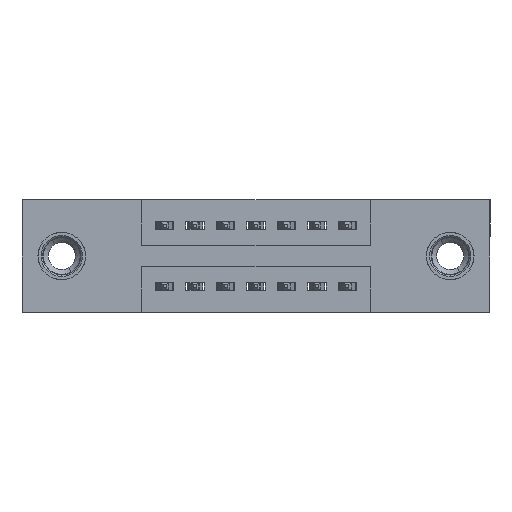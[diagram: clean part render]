
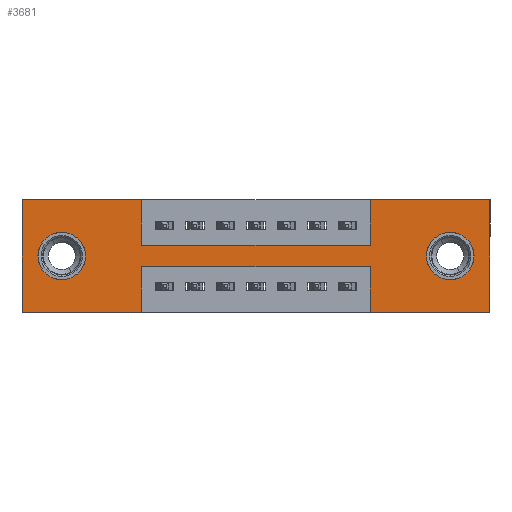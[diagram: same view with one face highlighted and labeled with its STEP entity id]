
A CAD part, front view. The second image highlights one B-rep face of the part: STEP entity #3681.
In plain terms, the highlighted planar face has unit normal (0, -1, 0).
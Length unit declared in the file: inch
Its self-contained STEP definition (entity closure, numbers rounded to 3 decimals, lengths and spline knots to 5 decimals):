
#15 = VERTEX_POINT ( 'NONE', #10215 ) ;
#115 = DIRECTION ( 'NONE',  ( 0., 0., -1. ) ) ;
#217 = ORIENTED_EDGE ( 'NONE', *, *, #5495, .T. ) ;
#316 = VERTEX_POINT ( 'NONE', #10917 ) ;
#375 = CARTESIAN_POINT ( 'NONE',  ( 1.405, 0., -0.263 ) ) ;
#463 = CARTESIAN_POINT ( 'NONE',  ( 0., 0., 0. ) ) ;
#607 = VECTOR ( 'NONE', #1782, 39.37008 ) ;
#608 = ORIENTED_EDGE ( 'NONE', *, *, #7334, .F. ) ;
#706 = PLANE ( 'NONE',  #6496 ) ;
#801 = DIRECTION ( 'NONE',  ( -1., 0., 0. ) ) ;
#875 = EDGE_CURVE ( 'NONE', #4007, #15, #11198, .T. ) ;
#892 = VERTEX_POINT ( 'NONE', #3567 ) ;
#929 = LINE ( 'NONE', #3808, #607 ) ;
#1279 = CARTESIAN_POINT ( 'NONE',  ( 0.3925, 0., -0.22 ) ) ;
#1328 = EDGE_LOOP ( 'NONE', ( #2870, #9219 ) ) ;
#1419 = LINE ( 'NONE', #4734, #11276 ) ;
#1485 = VERTEX_POINT ( 'NONE', #4570 ) ;
#1541 = ORIENTED_EDGE ( 'NONE', *, *, #5751, .F. ) ;
#1584 = EDGE_CURVE ( 'NONE', #15, #2349, #8369, .T. ) ;
#1629 = VERTEX_POINT ( 'NONE', #5442 ) ;
#1781 = DIRECTION ( 'NONE',  ( -1., 0., 0. ) ) ;
#1782 = DIRECTION ( 'NONE',  ( 0., 0., -1. ) ) ;
#2278 = EDGE_CURVE ( 'NONE', #892, #4111, #9325, .T. ) ;
#2349 = VERTEX_POINT ( 'NONE', #6331 ) ;
#2431 = VERTEX_POINT ( 'NONE', #5845 ) ;
#2599 = DIRECTION ( 'NONE',  ( 1., 0., 0. ) ) ;
#2659 = LINE ( 'NONE', #9602, #10525 ) ;
#2749 = VERTEX_POINT ( 'NONE', #1279 ) ;
#2765 = CARTESIAN_POINT ( 'NONE',  ( 0., 0., -0.37 ) ) ;
#2800 = DIRECTION ( 'NONE',  ( 0., 0., 1. ) ) ;
#2870 = ORIENTED_EDGE ( 'NONE', *, *, #9489, .T. ) ;
#3197 = EDGE_CURVE ( 'NONE', #8012, #2749, #6570, .T. ) ;
#3241 = CARTESIAN_POINT ( 'NONE',  ( 0.13, 0., -0.185 ) ) ;
#3267 = EDGE_LOOP ( 'NONE', ( #5348, #217 ) ) ;
#3363 = ORIENTED_EDGE ( 'NONE', *, *, #3197, .F. ) ;
#3415 = VECTOR ( 'NONE', #2599, 39.37008 ) ;
#3567 = CARTESIAN_POINT ( 'NONE',  ( 1.405, 0., -0.107 ) ) ;
#3649 = AXIS2_PLACEMENT_3D ( 'NONE', #6778, #6740, #6718 ) ;
#3681 = ADVANCED_FACE ( 'NONE', ( #6557, #6244, #4230 ), #706, .T. ) ;
#3697 = EDGE_CURVE ( 'NONE', #2749, #1485, #929, .T. ) ;
#3753 = AXIS2_PLACEMENT_3D ( 'NONE', #9921, #4281, #10851 ) ;
#3808 = CARTESIAN_POINT ( 'NONE',  ( 0.3925, 0., -0.37 ) ) ;
#4007 = VERTEX_POINT ( 'NONE', #10829 ) ;
#4111 = VERTEX_POINT ( 'NONE', #375 ) ;
#4114 = EDGE_CURVE ( 'NONE', #5319, #4868, #11682, .T. ) ;
#4216 = DIRECTION ( 'NONE',  ( 0., 0., 1. ) ) ;
#4230 = FACE_OUTER_BOUND ( 'NONE', #4938, .T. ) ;
#4281 = DIRECTION ( 'NONE',  ( 0., 1., 0. ) ) ;
#4471 = ORIENTED_EDGE ( 'NONE', *, *, #10329, .F. ) ;
#4570 = CARTESIAN_POINT ( 'NONE',  ( 0.3925, 0., -0.37 ) ) ;
#4626 = ORIENTED_EDGE ( 'NONE', *, *, #875, .F. ) ;
#4734 = CARTESIAN_POINT ( 'NONE',  ( 0., 0., -0.37 ) ) ;
#4776 = CARTESIAN_POINT ( 'NONE',  ( 1.405, 0., -0.185 ) ) ;
#4868 = VERTEX_POINT ( 'NONE', #9271 ) ;
#4908 = DIRECTION ( 'NONE',  ( 0., 0., -1. ) ) ;
#4938 = EDGE_LOOP ( 'NONE', ( #10666, #3363, #4471, #608, #1541, #10652, #8633, #7625, #6540, #11310, #4626, #6871 ) ) ;
#5319 = VERTEX_POINT ( 'NONE', #8257 ) ;
#5348 = ORIENTED_EDGE ( 'NONE', *, *, #2278, .T. ) ;
#5442 = CARTESIAN_POINT ( 'NONE',  ( 0.13, 0., -0.263 ) ) ;
#5495 = EDGE_CURVE ( 'NONE', #4111, #892, #7270, .T. ) ;
#5540 = EDGE_CURVE ( 'NONE', #1485, #4007, #9133, .T. ) ;
#5692 = LINE ( 'NONE', #8409, #3415 ) ;
#5721 = DIRECTION ( 'NONE',  ( 0., 0., -1. ) ) ;
#5751 = EDGE_CURVE ( 'NONE', #4868, #2431, #9526, .T. ) ;
#5774 = DIRECTION ( 'NONE',  ( 0., 0., -1. ) ) ;
#5845 = CARTESIAN_POINT ( 'NONE',  ( 1.535, 0., -0.37 ) ) ;
#6244 = FACE_BOUND ( 'NONE', #1328, .T. ) ;
#6318 = VECTOR ( 'NONE', #7145, 39.37008 ) ;
#6321 = CARTESIAN_POINT ( 'NONE',  ( 0.13, 0., -0.107 ) ) ;
#6331 = CARTESIAN_POINT ( 'NONE',  ( 0.3925, 0., 0. ) ) ;
#6376 = CARTESIAN_POINT ( 'NONE',  ( 0., 0., 0. ) ) ;
#6496 = AXIS2_PLACEMENT_3D ( 'NONE', #2765, #11285, #5721 ) ;
#6540 = ORIENTED_EDGE ( 'NONE', *, *, #9194, .F. ) ;
#6541 = VECTOR ( 'NONE', #9179, 39.37008 ) ;
#6548 = CIRCLE ( 'NONE', #9100, 0.078 ) ;
#6557 = FACE_BOUND ( 'NONE', #3267, .T. ) ;
#6570 = LINE ( 'NONE', #11350, #11141 ) ;
#6718 = DIRECTION ( 'NONE',  ( 0., 0., -1. ) ) ;
#6740 = DIRECTION ( 'NONE',  ( 0., 1., 0. ) ) ;
#6778 = CARTESIAN_POINT ( 'NONE',  ( 1.405, 0., -0.185 ) ) ;
#6788 = VERTEX_POINT ( 'NONE', #7909 ) ;
#6816 = VECTOR ( 'NONE', #115, 39.37008 ) ;
#6871 = ORIENTED_EDGE ( 'NONE', *, *, #5540, .F. ) ;
#7087 = CARTESIAN_POINT ( 'NONE',  ( 1.535, 0., 0. ) ) ;
#7129 = DIRECTION ( 'NONE',  ( 1., 0., 0. ) ) ;
#7145 = DIRECTION ( 'NONE',  ( 0., 0., 1. ) ) ;
#7270 = CIRCLE ( 'NONE', #8255, 0.078 ) ;
#7334 = EDGE_CURVE ( 'NONE', #2431, #11543, #1419, .T. ) ;
#7450 = CARTESIAN_POINT ( 'NONE',  ( 0., 0., 0. ) ) ;
#7596 = EDGE_CURVE ( 'NONE', #1629, #8356, #6548, .T. ) ;
#7609 = CARTESIAN_POINT ( 'NONE',  ( 1.1425, 0., -0.37 ) ) ;
#7625 = ORIENTED_EDGE ( 'NONE', *, *, #10188, .F. ) ;
#7863 = EDGE_CURVE ( 'NONE', #316, #5319, #10398, .T. ) ;
#7909 = CARTESIAN_POINT ( 'NONE',  ( 0.3925, 0., -0.15 ) ) ;
#8012 = VERTEX_POINT ( 'NONE', #9584 ) ;
#8255 = AXIS2_PLACEMENT_3D ( 'NONE', #4776, #11321, #5774 ) ;
#8257 = CARTESIAN_POINT ( 'NONE',  ( 1.1425, 0., 0. ) ) ;
#8356 = VERTEX_POINT ( 'NONE', #6321 ) ;
#8369 = LINE ( 'NONE', #7450, #10752 ) ;
#8409 = CARTESIAN_POINT ( 'NONE',  ( 0.3925, 0., -0.15 ) ) ;
#8482 = DIRECTION ( 'NONE',  ( 0., 0., 1. ) ) ;
#8633 = ORIENTED_EDGE ( 'NONE', *, *, #7863, .F. ) ;
#8960 = VECTOR ( 'NONE', #2800, 39.37008 ) ;
#9100 = AXIS2_PLACEMENT_3D ( 'NONE', #3241, #9862, #4216 ) ;
#9133 = LINE ( 'NONE', #11359, #11532 ) ;
#9179 = DIRECTION ( 'NONE',  ( 1., 0., 0. ) ) ;
#9194 = EDGE_CURVE ( 'NONE', #2349, #6788, #2659, .T. ) ;
#9219 = ORIENTED_EDGE ( 'NONE', *, *, #7596, .T. ) ;
#9227 = LINE ( 'NONE', #12167, #8960 ) ;
#9271 = CARTESIAN_POINT ( 'NONE',  ( 1.535, 0., 0. ) ) ;
#9325 = CIRCLE ( 'NONE', #3649, 0.078 ) ;
#9489 = EDGE_CURVE ( 'NONE', #8356, #1629, #11373, .T. ) ;
#9526 = LINE ( 'NONE', #7087, #6816 ) ;
#9584 = CARTESIAN_POINT ( 'NONE',  ( 1.1425, 0., -0.22 ) ) ;
#9602 = CARTESIAN_POINT ( 'NONE',  ( 0.3925, 0., 0. ) ) ;
#9862 = DIRECTION ( 'NONE',  ( 0., 1., 0. ) ) ;
#9921 = CARTESIAN_POINT ( 'NONE',  ( 0.13, 0., -0.185 ) ) ;
#10104 = VECTOR ( 'NONE', #8482, 39.37008 ) ;
#10188 = EDGE_CURVE ( 'NONE', #6788, #316, #5692, .T. ) ;
#10215 = CARTESIAN_POINT ( 'NONE',  ( 0., 0., 0. ) ) ;
#10259 = CARTESIAN_POINT ( 'NONE',  ( 1.1425, 0., 0. ) ) ;
#10329 = EDGE_CURVE ( 'NONE', #11543, #8012, #9227, .T. ) ;
#10398 = LINE ( 'NONE', #10259, #10104 ) ;
#10525 = VECTOR ( 'NONE', #4908, 39.37008 ) ;
#10652 = ORIENTED_EDGE ( 'NONE', *, *, #4114, .F. ) ;
#10666 = ORIENTED_EDGE ( 'NONE', *, *, #3697, .F. ) ;
#10752 = VECTOR ( 'NONE', #7129, 39.37008 ) ;
#10829 = CARTESIAN_POINT ( 'NONE',  ( 0., 0., -0.37 ) ) ;
#10851 = DIRECTION ( 'NONE',  ( 0., 0., 1. ) ) ;
#10917 = CARTESIAN_POINT ( 'NONE',  ( 1.1425, 0., -0.15 ) ) ;
#11141 = VECTOR ( 'NONE', #11385, 39.37008 ) ;
#11198 = LINE ( 'NONE', #463, #6318 ) ;
#11276 = VECTOR ( 'NONE', #1781, 39.37008 ) ;
#11285 = DIRECTION ( 'NONE',  ( 0., -1., 0. ) ) ;
#11310 = ORIENTED_EDGE ( 'NONE', *, *, #1584, .F. ) ;
#11321 = DIRECTION ( 'NONE',  ( 0., 1., 0. ) ) ;
#11350 = CARTESIAN_POINT ( 'NONE',  ( 0.3925, 0., -0.22 ) ) ;
#11359 = CARTESIAN_POINT ( 'NONE',  ( 0., 0., -0.37 ) ) ;
#11373 = CIRCLE ( 'NONE', #3753, 0.078 ) ;
#11385 = DIRECTION ( 'NONE',  ( -1., 0., 0. ) ) ;
#11532 = VECTOR ( 'NONE', #801, 39.37008 ) ;
#11543 = VERTEX_POINT ( 'NONE', #7609 ) ;
#11682 = LINE ( 'NONE', #6376, #6541 ) ;
#12167 = CARTESIAN_POINT ( 'NONE',  ( 1.1425, 0., -0.37 ) ) ;
